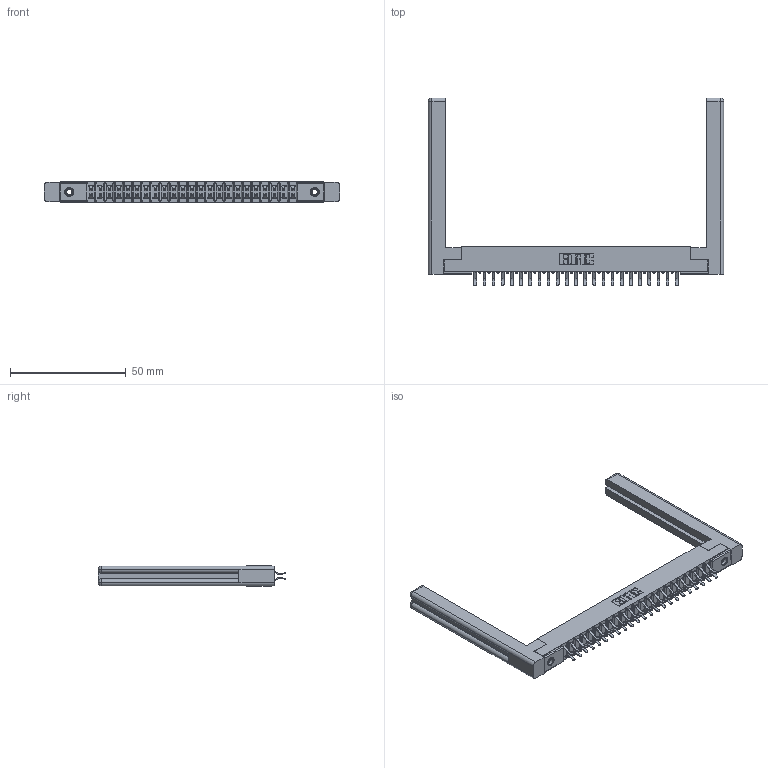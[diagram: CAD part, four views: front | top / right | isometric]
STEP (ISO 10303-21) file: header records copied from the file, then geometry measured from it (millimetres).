
FILE_DESCRIPTION (( 'STEP AP203' ), '1' );
FILE_NAME ('307-046-456-258.STEP', '2020-09-30T02:46:35', ( '' ), ( '' ), 'SwSTEP 2.0', 'SolidWorks 2020', '' );
FILE_SCHEMA (( 'CONFIG_CONTROL_DESIGN' ));
Length unit declared in the file: inch
Products named in the file (5): 345-250-001_345-250-001-102; 307-046-456-258; 307 Part_.156 Dia Mounting Holes; 307-220-058; 307-290-001_556
Assembly tree (51 placements, depth 2):
  307-046-456-258
    307 Part_.156 Dia Mounting Holes
    307-290-001_556  x46
    307-220-058  x2
    345-250-001_345-250-001-102  x2
Bounding box: 127.76 x 81.28 x 8.71 mm (x, y, z)
Volume: 16035.2 mm3; surface area: 19841.2 mm2
Topology: 51 solids, 51 shells, 2584 faces, 7209 edges, 4666 vertices
Faces by surface type: plane 1672, cylinder 840, sphere 48, torus 12, cone 12
Entity records: 25533 total; most frequent: CARTESIAN_POINT 4202, ORIENTED_EDGE 4104, DIRECTION 4082, EDGE_CURVE 2052, VECTOR 1562, LINE 1562, VERTEX_POINT 1326, AXIS2_PLACEMENT_3D 1260
